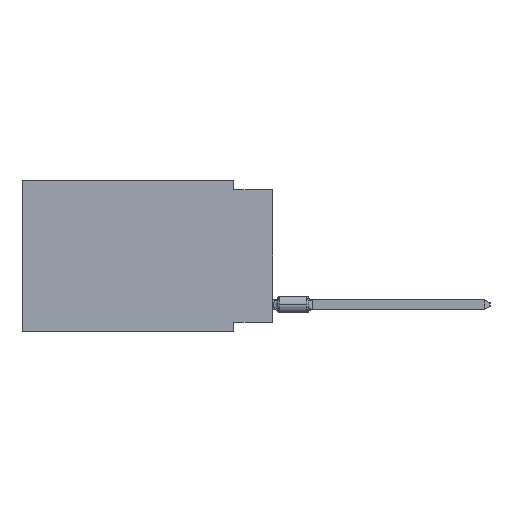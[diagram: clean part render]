
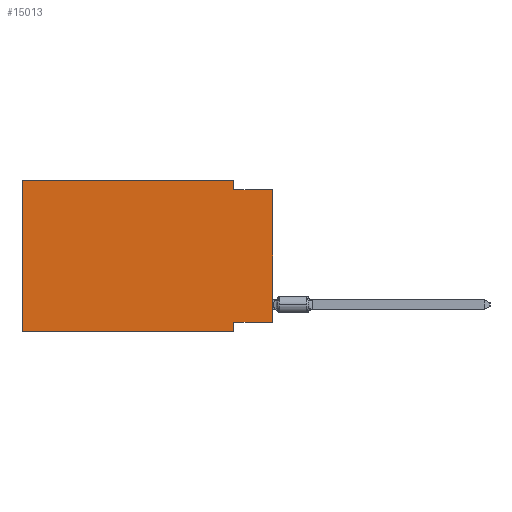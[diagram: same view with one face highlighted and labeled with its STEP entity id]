
A CAD part, left-side view. The second image highlights one B-rep face of the part: STEP entity #15013.
In plain terms, the highlighted planar face has unit normal (-1, 0, 0).
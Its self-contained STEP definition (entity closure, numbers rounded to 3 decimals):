
#1676 = ORIENTED_EDGE ( 'NONE', *, *, #14341, .F. ) ;
#1731 = CARTESIAN_POINT ( 'NONE',  ( 0., 16.383, 0. ) ) ;
#2254 = ORIENTED_EDGE ( 'NONE', *, *, #34743, .F. ) ;
#2255 = CARTESIAN_POINT ( 'NONE',  ( 0., 16.383, 0. ) ) ;
#2270 = VECTOR ( 'NONE', #29999, 1000. ) ;
#4081 = LINE ( 'NONE', #29563, #2270 ) ;
#5932 = LINE ( 'NONE', #13399, #60794 ) ;
#6594 = CARTESIAN_POINT ( 'NONE',  ( 0., 2.54, -0.635 ) ) ;
#6933 = VERTEX_POINT ( 'NONE', #82314 ) ;
#7335 = CARTESIAN_POINT ( 'NONE',  ( 0., 16.383, 0. ) ) ;
#8082 = CARTESIAN_POINT ( 'NONE',  ( 0., 0., -9.271 ) ) ;
#8410 = CARTESIAN_POINT ( 'NONE',  ( 0., 0., -9.271 ) ) ;
#11780 = VECTOR ( 'NONE', #36047, 1000. ) ;
#12799 = LINE ( 'NONE', #19386, #38805 ) ;
#13399 = CARTESIAN_POINT ( 'NONE',  ( 0., 2.54, 0. ) ) ;
#13778 = VECTOR ( 'NONE', #78557, 1000. ) ;
#14341 = EDGE_CURVE ( 'NONE', #69017, #66327, #68511, .T. ) ;
#15013 = ADVANCED_FACE ( 'NONE', ( #74031 ), #81021, .F. ) ;
#15201 = ORIENTED_EDGE ( 'NONE', *, *, #72258, .T. ) ;
#15596 = EDGE_LOOP ( 'NONE', ( #15201, #53910, #21237, #31178, #2254, #31481, #64759, #1676 ) ) ;
#17630 = CARTESIAN_POINT ( 'NONE',  ( 0., 16.383, -9.906 ) ) ;
#18475 = LINE ( 'NONE', #84713, #13778 ) ;
#19386 = CARTESIAN_POINT ( 'NONE',  ( 0., 2.54, -9.906 ) ) ;
#20852 = CARTESIAN_POINT ( 'NONE',  ( 0., 16.383, 0. ) ) ;
#21237 = ORIENTED_EDGE ( 'NONE', *, *, #65840, .F. ) ;
#21560 = DIRECTION ( 'NONE',  ( 0., 0., 1. ) ) ;
#22087 = VERTEX_POINT ( 'NONE', #6594 ) ;
#23964 = CARTESIAN_POINT ( 'NONE',  ( 0., 2.54, 0. ) ) ;
#26055 = LINE ( 'NONE', #58950, #78770 ) ;
#27540 = EDGE_CURVE ( 'NONE', #66327, #6933, #12799, .T. ) ;
#29563 = CARTESIAN_POINT ( 'NONE',  ( 0., 0., 0. ) ) ;
#29999 = DIRECTION ( 'NONE',  ( 0., 0., 1. ) ) ;
#30536 = VERTEX_POINT ( 'NONE', #1731 ) ;
#31178 = ORIENTED_EDGE ( 'NONE', *, *, #53136, .F. ) ;
#31481 = ORIENTED_EDGE ( 'NONE', *, *, #54922, .T. ) ;
#32086 = VECTOR ( 'NONE', #69931, 1000. ) ;
#33575 = DIRECTION ( 'NONE',  ( 0., 0., -1. ) ) ;
#34100 = DIRECTION ( 'NONE',  ( 0., 0., -1. ) ) ;
#34743 = EDGE_CURVE ( 'NONE', #55254, #30536, #75058, .T. ) ;
#35507 = CARTESIAN_POINT ( 'NONE',  ( 0., 0., -0.635 ) ) ;
#35688 = AXIS2_PLACEMENT_3D ( 'NONE', #7335, #39384, #34100 ) ;
#36047 = DIRECTION ( 'NONE',  ( 0., 1., 0. ) ) ;
#38805 = VECTOR ( 'NONE', #80338, 1000. ) ;
#39384 = DIRECTION ( 'NONE',  ( 1., 0., 0. ) ) ;
#39780 = VERTEX_POINT ( 'NONE', #35507 ) ;
#42474 = EDGE_CURVE ( 'NONE', #22087, #39780, #18475, .T. ) ;
#49304 = VERTEX_POINT ( 'NONE', #23964 ) ;
#52681 = CARTESIAN_POINT ( 'NONE',  ( 0., 2.54, -9.271 ) ) ;
#53136 = EDGE_CURVE ( 'NONE', #30536, #49304, #80923, .T. ) ;
#53910 = ORIENTED_EDGE ( 'NONE', *, *, #42474, .F. ) ;
#54922 = EDGE_CURVE ( 'NONE', #55254, #6933, #26055, .T. ) ;
#55254 = VERTEX_POINT ( 'NONE', #17630 ) ;
#58950 = CARTESIAN_POINT ( 'NONE',  ( 0., 16.383, -9.906 ) ) ;
#59251 = VECTOR ( 'NONE', #21560, 1000. ) ;
#60794 = VECTOR ( 'NONE', #33575, 1000. ) ;
#64759 = ORIENTED_EDGE ( 'NONE', *, *, #27540, .F. ) ;
#65840 = EDGE_CURVE ( 'NONE', #49304, #22087, #5932, .T. ) ;
#65960 = DIRECTION ( 'NONE',  ( 0., -1., 0. ) ) ;
#66327 = VERTEX_POINT ( 'NONE', #52681 ) ;
#68511 = LINE ( 'NONE', #8410, #11780 ) ;
#69017 = VERTEX_POINT ( 'NONE', #8082 ) ;
#69931 = DIRECTION ( 'NONE',  ( 0., -1., 0. ) ) ;
#72258 = EDGE_CURVE ( 'NONE', #69017, #39780, #4081, .T. ) ;
#74031 = FACE_OUTER_BOUND ( 'NONE', #15596, .T. ) ;
#75058 = LINE ( 'NONE', #2255, #59251 ) ;
#78557 = DIRECTION ( 'NONE',  ( 0., -1., 0. ) ) ;
#78770 = VECTOR ( 'NONE', #65960, 1000. ) ;
#80338 = DIRECTION ( 'NONE',  ( 0., 0., -1. ) ) ;
#80923 = LINE ( 'NONE', #20852, #32086 ) ;
#81021 = PLANE ( 'NONE',  #35688 ) ;
#82314 = CARTESIAN_POINT ( 'NONE',  ( 0., 2.54, -9.906 ) ) ;
#84713 = CARTESIAN_POINT ( 'NONE',  ( 0., 0., -0.635 ) ) ;
